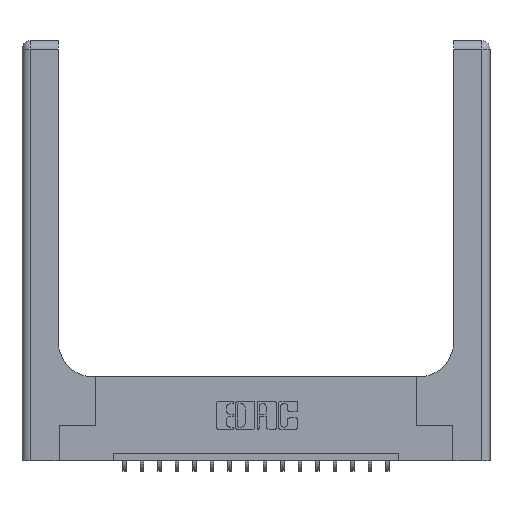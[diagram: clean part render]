
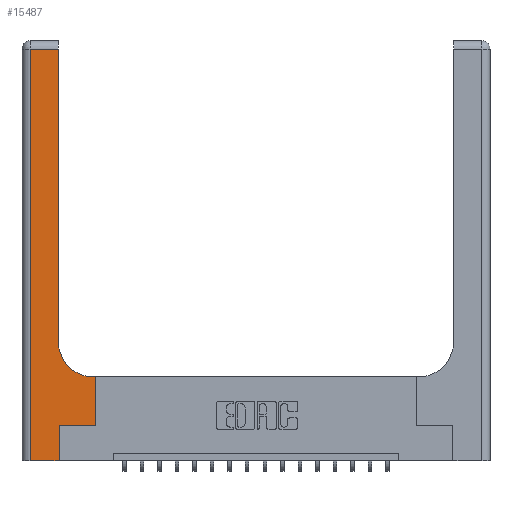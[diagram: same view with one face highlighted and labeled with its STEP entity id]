
A CAD part, top view. The second image highlights one B-rep face of the part: STEP entity #15487.
In plain terms, the highlighted planar face has unit normal (0, 0, 1).
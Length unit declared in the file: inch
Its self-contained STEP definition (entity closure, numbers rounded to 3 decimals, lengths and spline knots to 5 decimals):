
#1079 = ORIENTED_EDGE ( 'NONE', *, *, #5137, .T. ) ;
#1873 = VERTEX_POINT ( 'NONE', #4660 ) ;
#2035 = DIRECTION ( 'NONE',  ( 0., 1., 0. ) ) ;
#2258 = LINE ( 'NONE', #8308, #4537 ) ;
#2290 = LINE ( 'NONE', #13913, #6797 ) ;
#2388 = EDGE_CURVE ( 'NONE', #1873, #14506, #9309, .T. ) ;
#2526 = CARTESIAN_POINT ( 'NONE',  ( 0.265, 0., 0.37 ) ) ;
#3100 = ORIENTED_EDGE ( 'NONE', *, *, #18205, .T. ) ;
#3542 = DIRECTION ( 'NONE',  ( 0., 0., -1. ) ) ;
#3616 = VERTEX_POINT ( 'NONE', #18236 ) ;
#3636 = EDGE_CURVE ( 'NONE', #4685, #11336, #9315, .T. ) ;
#3825 = CARTESIAN_POINT ( 'NONE',  ( 0.26, 0.85, 0.37 ) ) ;
#4142 = LINE ( 'NONE', #19032, #7786 ) ;
#4154 = DIRECTION ( 'NONE',  ( -1., 0., 0. ) ) ;
#4443 = CARTESIAN_POINT ( 'NONE',  ( 0.51, 0.6, 0.37 ) ) ;
#4537 = VECTOR ( 'NONE', #4154, 39.37008 ) ;
#4660 = CARTESIAN_POINT ( 'NONE',  ( 0.528, 0.25, 0.37 ) ) ;
#4685 = VERTEX_POINT ( 'NONE', #4443 ) ;
#4739 = EDGE_LOOP ( 'NONE', ( #9598, #10451, #1079, #12186, #11688, #10977, #5766, #3100, #18611 ) ) ;
#4988 = DIRECTION ( 'NONE',  ( -1., 0., 0. ) ) ;
#5137 = EDGE_CURVE ( 'NONE', #13694, #3616, #2290, .T. ) ;
#5695 = LINE ( 'NONE', #7081, #6140 ) ;
#5766 = ORIENTED_EDGE ( 'NONE', *, *, #2388, .T. ) ;
#6128 = CARTESIAN_POINT ( 'NONE',  ( 0.528, 0.25, 0.37 ) ) ;
#6140 = VECTOR ( 'NONE', #12969, 39.37008 ) ;
#6300 = LINE ( 'NONE', #13850, #18506 ) ;
#6444 = CARTESIAN_POINT ( 'NONE',  ( 0., 3., 0.37 ) ) ;
#6553 = DIRECTION ( 'NONE',  ( 0., -1., 0. ) ) ;
#6794 = EDGE_CURVE ( 'NONE', #3616, #16428, #12144, .T. ) ;
#6797 = VECTOR ( 'NONE', #6553, 39.37008 ) ;
#7081 = CARTESIAN_POINT ( 'NONE',  ( 0.265, 0.25, 0.37 ) ) ;
#7786 = VECTOR ( 'NONE', #11518, 39.37008 ) ;
#8308 = CARTESIAN_POINT ( 'NONE',  ( 0., 2.94, 0.37 ) ) ;
#8351 = AXIS2_PLACEMENT_3D ( 'NONE', #13802, #11962, #9147 ) ;
#8409 = DIRECTION ( 'NONE',  ( 0., 1., 0. ) ) ;
#8652 = CARTESIAN_POINT ( 'NONE',  ( 0.265, 0., 0.37 ) ) ;
#9146 = EDGE_CURVE ( 'NONE', #18557, #13694, #2258, .T. ) ;
#9147 = DIRECTION ( 'NONE',  ( 1., 0., 0. ) ) ;
#9167 = EDGE_CURVE ( 'NONE', #16428, #18954, #17214, .T. ) ;
#9250 = FACE_OUTER_BOUND ( 'NONE', #4739, .T. ) ;
#9309 = LINE ( 'NONE', #6128, #13310 ) ;
#9315 = CIRCLE ( 'NONE', #8351, 0.25 ) ;
#9598 = ORIENTED_EDGE ( 'NONE', *, *, #13258, .T. ) ;
#10302 = VECTOR ( 'NONE', #17739, 39.37008 ) ;
#10451 = ORIENTED_EDGE ( 'NONE', *, *, #9146, .T. ) ;
#10977 = ORIENTED_EDGE ( 'NONE', *, *, #12450, .T. ) ;
#11315 = VECTOR ( 'NONE', #8409, 39.37008 ) ;
#11336 = VERTEX_POINT ( 'NONE', #3825 ) ;
#11479 = AXIS2_PLACEMENT_3D ( 'NONE', #6444, #3542, #4988 ) ;
#11518 = DIRECTION ( 'NONE',  ( -1., 0., 0. ) ) ;
#11537 = CARTESIAN_POINT ( 'NONE',  ( 0.528, 0.6, 0.37 ) ) ;
#11688 = ORIENTED_EDGE ( 'NONE', *, *, #9167, .T. ) ;
#11962 = DIRECTION ( 'NONE',  ( 0., 0., -1. ) ) ;
#12033 = DIRECTION ( 'NONE',  ( 0., 1., 0. ) ) ;
#12144 = LINE ( 'NONE', #12241, #10302 ) ;
#12186 = ORIENTED_EDGE ( 'NONE', *, *, #6794, .T. ) ;
#12241 = CARTESIAN_POINT ( 'NONE',  ( 0., 0., 0.37 ) ) ;
#12450 = EDGE_CURVE ( 'NONE', #18954, #1873, #5695, .T. ) ;
#12969 = DIRECTION ( 'NONE',  ( 1., 0., 0. ) ) ;
#13258 = EDGE_CURVE ( 'NONE', #11336, #18557, #6300, .T. ) ;
#13310 = VECTOR ( 'NONE', #12033, 39.37008 ) ;
#13694 = VERTEX_POINT ( 'NONE', #17637 ) ;
#13802 = CARTESIAN_POINT ( 'NONE',  ( 0.51, 0.85, 0.37 ) ) ;
#13807 = PLANE ( 'NONE',  #11479 ) ;
#13850 = CARTESIAN_POINT ( 'NONE',  ( 0.26, 3., 0.37 ) ) ;
#13913 = CARTESIAN_POINT ( 'NONE',  ( 0.06, 3., 0.37 ) ) ;
#14506 = VERTEX_POINT ( 'NONE', #11537 ) ;
#15487 = ADVANCED_FACE ( 'NONE', ( #9250 ), #13807, .F. ) ;
#16428 = VERTEX_POINT ( 'NONE', #8652 ) ;
#17055 = CARTESIAN_POINT ( 'NONE',  ( 0.265, 0.25, 0.37 ) ) ;
#17214 = LINE ( 'NONE', #2526, #11315 ) ;
#17637 = CARTESIAN_POINT ( 'NONE',  ( 0.06, 2.94, 0.37 ) ) ;
#17739 = DIRECTION ( 'NONE',  ( 1., 0., 0. ) ) ;
#18205 = EDGE_CURVE ( 'NONE', #14506, #4685, #4142, .T. ) ;
#18236 = CARTESIAN_POINT ( 'NONE',  ( 0.06, 0., 0.37 ) ) ;
#18367 = CARTESIAN_POINT ( 'NONE',  ( 0.26, 2.94, 0.37 ) ) ;
#18506 = VECTOR ( 'NONE', #2035, 39.37008 ) ;
#18557 = VERTEX_POINT ( 'NONE', #18367 ) ;
#18611 = ORIENTED_EDGE ( 'NONE', *, *, #3636, .T. ) ;
#18954 = VERTEX_POINT ( 'NONE', #17055 ) ;
#19032 = CARTESIAN_POINT ( 'NONE',  ( 0.26, 0.6, 0.37 ) ) ;
